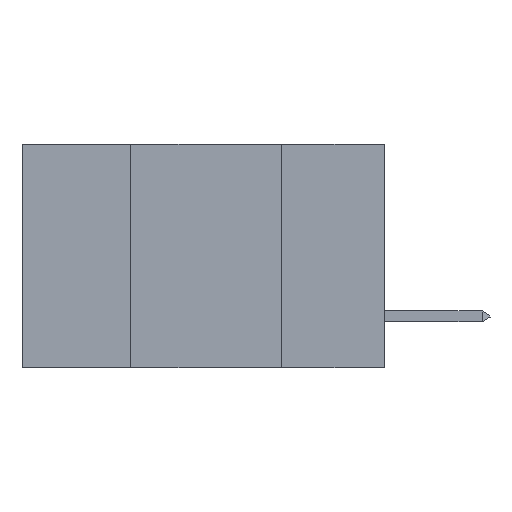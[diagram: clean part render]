
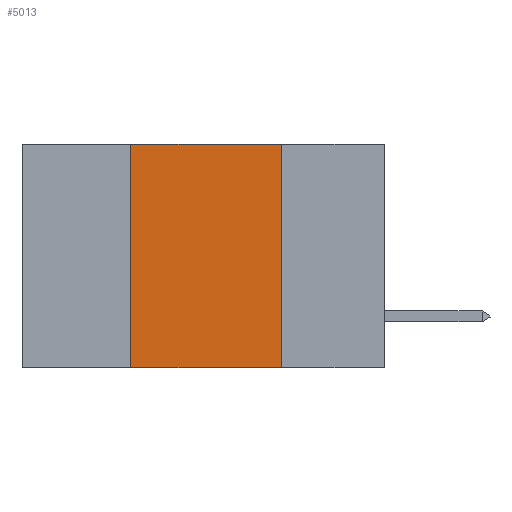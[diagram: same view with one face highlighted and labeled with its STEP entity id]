
A CAD part, left-side view. The second image highlights one B-rep face of the part: STEP entity #5013.
In plain terms, the highlighted planar face has unit normal (-1, 0, 0).
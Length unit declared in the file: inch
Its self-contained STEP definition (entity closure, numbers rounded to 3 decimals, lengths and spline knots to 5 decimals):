
#752 = DIRECTION ( 'NONE',  ( 0., 0., -1. ) ) ;
#784 = CARTESIAN_POINT ( 'NONE',  ( 0., 0.42, -0.37 ) ) ;
#904 = VECTOR ( 'NONE', #2565, 39.37008 ) ;
#2565 = DIRECTION ( 'NONE',  ( 0., 0., -1. ) ) ;
#2978 = VECTOR ( 'NONE', #4448, 39.37008 ) ;
#4448 = DIRECTION ( 'NONE',  ( 0., -1., 0. ) ) ;
#4507 = CARTESIAN_POINT ( 'NONE',  ( 0., 0.17, -0.37 ) ) ;
#5013 = ADVANCED_FACE ( 'NONE', ( #5836 ), #23636, .F. ) ;
#5836 = FACE_OUTER_BOUND ( 'NONE', #16760, .T. ) ;
#6694 = VERTEX_POINT ( 'NONE', #4507 ) ;
#7740 = ORIENTED_EDGE ( 'NONE', *, *, #18968, .F. ) ;
#7807 = ORIENTED_EDGE ( 'NONE', *, *, #13655, .T. ) ;
#8364 = CARTESIAN_POINT ( 'NONE',  ( 0., 0.17, 0. ) ) ;
#8789 = DIRECTION ( 'NONE',  ( 0., 0., 1. ) ) ;
#9432 = VERTEX_POINT ( 'NONE', #10769 ) ;
#9448 = VERTEX_POINT ( 'NONE', #784 ) ;
#9770 = AXIS2_PLACEMENT_3D ( 'NONE', #18147, #13900, #752 ) ;
#10137 = LINE ( 'NONE', #20179, #14046 ) ;
#10148 = CARTESIAN_POINT ( 'NONE',  ( 0., 0.17, 0. ) ) ;
#10769 = CARTESIAN_POINT ( 'NONE',  ( 0., 0.42, 0. ) ) ;
#11180 = ORIENTED_EDGE ( 'NONE', *, *, #22157, .F. ) ;
#13409 = LINE ( 'NONE', #20573, #17646 ) ;
#13655 = EDGE_CURVE ( 'NONE', #9448, #6694, #10137, .T. ) ;
#13900 = DIRECTION ( 'NONE',  ( 1., 0., 0. ) ) ;
#14046 = VECTOR ( 'NONE', #23531, 39.37008 ) ;
#14126 = LINE ( 'NONE', #22211, #2978 ) ;
#14983 = ORIENTED_EDGE ( 'NONE', *, *, #19689, .F. ) ;
#15121 = LINE ( 'NONE', #8364, #904 ) ;
#16760 = EDGE_LOOP ( 'NONE', ( #7740, #14983, #11180, #7807 ) ) ;
#17646 = VECTOR ( 'NONE', #8789, 39.37008 ) ;
#18147 = CARTESIAN_POINT ( 'NONE',  ( 0., 0.6, 0. ) ) ;
#18968 = EDGE_CURVE ( 'NONE', #23019, #6694, #15121, .T. ) ;
#19689 = EDGE_CURVE ( 'NONE', #9432, #23019, #14126, .T. ) ;
#20179 = CARTESIAN_POINT ( 'NONE',  ( 0., 0.6, -0.37 ) ) ;
#20573 = CARTESIAN_POINT ( 'NONE',  ( 0., 0.42, 0. ) ) ;
#22157 = EDGE_CURVE ( 'NONE', #9448, #9432, #13409, .T. ) ;
#22211 = CARTESIAN_POINT ( 'NONE',  ( 0., 0.6, 0. ) ) ;
#23019 = VERTEX_POINT ( 'NONE', #10148 ) ;
#23531 = DIRECTION ( 'NONE',  ( 0., -1., 0. ) ) ;
#23636 = PLANE ( 'NONE',  #9770 ) ;
